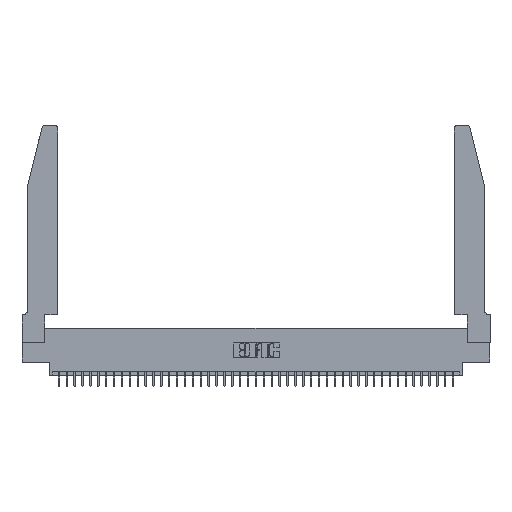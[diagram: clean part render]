
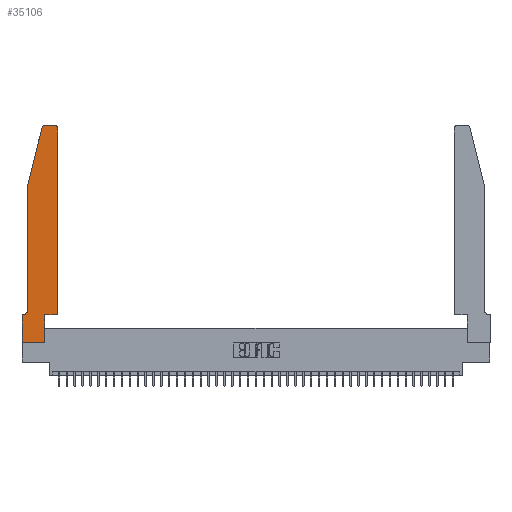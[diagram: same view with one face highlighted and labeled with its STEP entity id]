
A CAD part, top view. The second image highlights one B-rep face of the part: STEP entity #35106.
In plain terms, the highlighted planar face has unit normal (0, 0, 1).
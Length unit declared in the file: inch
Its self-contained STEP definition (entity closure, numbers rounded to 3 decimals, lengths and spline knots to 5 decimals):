
#385 = CARTESIAN_POINT ( 'NONE',  ( 0.2865, 0., 0.37 ) ) ;
#411 = CARTESIAN_POINT ( 'NONE',  ( 0.4205, 2.72, 0.37 ) ) ;
#520 = DIRECTION ( 'NONE',  ( 0., 0., 1. ) ) ;
#677 = EDGE_CURVE ( 'NONE', #34103, #35598, #38022, .T. ) ;
#1090 = EDGE_CURVE ( 'NONE', #5369, #17566, #35626, .T. ) ;
#2582 = DIRECTION ( 'NONE',  ( -1., 0., 0. ) ) ;
#2632 = DIRECTION ( 'NONE',  ( -1., 0., 0. ) ) ;
#3723 = CARTESIAN_POINT ( 'NONE',  ( 0.4505, 0.35, 0.37 ) ) ;
#3755 = VERTEX_POINT ( 'NONE', #10312 ) ;
#3899 = VECTOR ( 'NONE', #2582, 39.37008 ) ;
#3991 = ORIENTED_EDGE ( 'NONE', *, *, #20890, .T. ) ;
#4508 = CARTESIAN_POINT ( 'NONE',  ( 0.4505, 0.35, 0.37 ) ) ;
#4546 = EDGE_CURVE ( 'NONE', #33436, #18981, #41330, .T. ) ;
#5369 = VERTEX_POINT ( 'NONE', #385 ) ;
#5561 = LINE ( 'NONE', #32865, #16286 ) ;
#5621 = EDGE_CURVE ( 'NONE', #35598, #5369, #42918, .T. ) ;
#5652 = CARTESIAN_POINT ( 'NONE',  ( 0.0755, 2., 0.37 ) ) ;
#5817 = VECTOR ( 'NONE', #32319, 39.37008 ) ;
#5860 = VERTEX_POINT ( 'NONE', #25192 ) ;
#6333 = PLANE ( 'NONE',  #38865 ) ;
#6445 = CIRCLE ( 'NONE', #29824, 0.07 ) ;
#6705 = VECTOR ( 'NONE', #22979, 39.37008 ) ;
#7182 = VECTOR ( 'NONE', #7384, 39.37008 ) ;
#7300 = ORIENTED_EDGE ( 'NONE', *, *, #5621, .T. ) ;
#7384 = DIRECTION ( 'NONE',  ( 0., 1., 0. ) ) ;
#7824 = VECTOR ( 'NONE', #28045, 39.37008 ) ;
#8460 = DIRECTION ( 'NONE',  ( 1., 0., 0. ) ) ;
#8964 = ORIENTED_EDGE ( 'NONE', *, *, #19388, .T. ) ;
#9311 = VECTOR ( 'NONE', #20646, 39.37008 ) ;
#9791 = LINE ( 'NONE', #19997, #9311 ) ;
#10312 = CARTESIAN_POINT ( 'NONE',  ( 0.25487, 2.72718, 0.37 ) ) ;
#10356 = VERTEX_POINT ( 'NONE', #19273 ) ;
#11798 = LINE ( 'NONE', #25353, #39846 ) ;
#11948 = ORIENTED_EDGE ( 'NONE', *, *, #40208, .T. ) ;
#12158 = ORIENTED_EDGE ( 'NONE', *, *, #1090, .T. ) ;
#12592 = CARTESIAN_POINT ( 'NONE',  ( 0.0055, 0.42, 0.37 ) ) ;
#12982 = LINE ( 'NONE', #26535, #6705 ) ;
#14249 = DIRECTION ( 'NONE',  ( 1., 0., 0. ) ) ;
#14704 = CARTESIAN_POINT ( 'NONE',  ( 0., 0., 0.37 ) ) ;
#16005 = DIRECTION ( 'NONE',  ( -0.239, -0.971, 0. ) ) ;
#16286 = VECTOR ( 'NONE', #16005, 39.37008 ) ;
#17566 = VERTEX_POINT ( 'NONE', #32628 ) ;
#17764 = VECTOR ( 'NONE', #18122, 39.37008 ) ;
#18122 = DIRECTION ( 'NONE',  ( 0., 1., 0. ) ) ;
#18557 = ORIENTED_EDGE ( 'NONE', *, *, #677, .T. ) ;
#18661 = FACE_OUTER_BOUND ( 'NONE', #30110, .T. ) ;
#18782 = CARTESIAN_POINT ( 'NONE',  ( 0.2865, 0.35, 0.37 ) ) ;
#18981 = VERTEX_POINT ( 'NONE', #43020 ) ;
#19273 = CARTESIAN_POINT ( 'NONE',  ( 0.0755, 0.42, 0.37 ) ) ;
#19388 = EDGE_CURVE ( 'NONE', #10356, #26324, #6445, .T. ) ;
#19410 = CARTESIAN_POINT ( 'NONE',  ( 0.0755, 0.35, 0.37 ) ) ;
#19882 = CARTESIAN_POINT ( 'NONE',  ( 0., 0.35, 0.37 ) ) ;
#19997 = CARTESIAN_POINT ( 'NONE',  ( 0.2605, 2.75, 0.37 ) ) ;
#20646 = DIRECTION ( 'NONE',  ( -1., 0., 0. ) ) ;
#20683 = ORIENTED_EDGE ( 'NONE', *, *, #4546, .T. ) ;
#20890 = EDGE_CURVE ( 'NONE', #18981, #5860, #39754, .T. ) ;
#21616 = CARTESIAN_POINT ( 'NONE',  ( 0.284, 2.75, 0.37 ) ) ;
#22564 = EDGE_CURVE ( 'NONE', #17566, #33436, #11798, .T. ) ;
#22979 = DIRECTION ( 'NONE',  ( 0., -1., 0. ) ) ;
#23001 = AXIS2_PLACEMENT_3D ( 'NONE', #30895, #520, #14249 ) ;
#25192 = CARTESIAN_POINT ( 'NONE',  ( 0.4205, 2.75, 0.37 ) ) ;
#25353 = CARTESIAN_POINT ( 'NONE',  ( 0.4505, 0.35, 0.37 ) ) ;
#26324 = VERTEX_POINT ( 'NONE', #28444 ) ;
#26521 = CIRCLE ( 'NONE', #23001, 0.03 ) ;
#26535 = CARTESIAN_POINT ( 'NONE',  ( 0.0755, 2., 0.37 ) ) ;
#26592 = DIRECTION ( 'NONE',  ( 0., 0., -1. ) ) ;
#27272 = EDGE_CURVE ( 'NONE', #27278, #10356, #12982, .T. ) ;
#27278 = VERTEX_POINT ( 'NONE', #5652 ) ;
#27321 = EDGE_CURVE ( 'NONE', #26324, #34103, #35855, .T. ) ;
#28045 = DIRECTION ( 'NONE',  ( 0., -1., 0. ) ) ;
#28444 = CARTESIAN_POINT ( 'NONE',  ( 0.0055, 0.35, 0.37 ) ) ;
#29199 = CARTESIAN_POINT ( 'NONE',  ( 0., 0., 0.37 ) ) ;
#29824 = AXIS2_PLACEMENT_3D ( 'NONE', #12592, #26592, #2632 ) ;
#29977 = EDGE_CURVE ( 'NONE', #35822, #3755, #26521, .T. ) ;
#30088 = DIRECTION ( 'NONE',  ( 1., 0., 0. ) ) ;
#30110 = EDGE_LOOP ( 'NONE', ( #11948, #43516, #31095, #33142, #8964, #39483, #18557, #7300, #12158, #33891, #20683, #3991 ) ) ;
#30782 = DIRECTION ( 'NONE',  ( 1., 0., 0. ) ) ;
#30895 = CARTESIAN_POINT ( 'NONE',  ( 0.284, 2.72, 0.37 ) ) ;
#31095 = ORIENTED_EDGE ( 'NONE', *, *, #38767, .T. ) ;
#32319 = DIRECTION ( 'NONE',  ( 1., 0., 0. ) ) ;
#32628 = CARTESIAN_POINT ( 'NONE',  ( 0.2865, 0.35, 0.37 ) ) ;
#32865 = CARTESIAN_POINT ( 'NONE',  ( 0.0755, 2., 0.37 ) ) ;
#32919 = CARTESIAN_POINT ( 'NONE',  ( 0., 0.35, 0.37 ) ) ;
#33142 = ORIENTED_EDGE ( 'NONE', *, *, #27272, .T. ) ;
#33413 = DIRECTION ( 'NONE',  ( 0., 0., 1. ) ) ;
#33436 = VERTEX_POINT ( 'NONE', #3723 ) ;
#33891 = ORIENTED_EDGE ( 'NONE', *, *, #22564, .T. ) ;
#34103 = VERTEX_POINT ( 'NONE', #32919 ) ;
#34105 = DIRECTION ( 'NONE',  ( 0., 0., 1. ) ) ;
#35106 = ADVANCED_FACE ( 'NONE', ( #18661 ), #6333, .T. ) ;
#35598 = VERTEX_POINT ( 'NONE', #36030 ) ;
#35626 = LINE ( 'NONE', #18782, #17764 ) ;
#35822 = VERTEX_POINT ( 'NONE', #21616 ) ;
#35855 = LINE ( 'NONE', #19410, #3899 ) ;
#36030 = CARTESIAN_POINT ( 'NONE',  ( 0., 0., 0.37 ) ) ;
#38022 = LINE ( 'NONE', #14704, #7824 ) ;
#38767 = EDGE_CURVE ( 'NONE', #3755, #27278, #5561, .T. ) ;
#38865 = AXIS2_PLACEMENT_3D ( 'NONE', #19882, #33413, #30088 ) ;
#39483 = ORIENTED_EDGE ( 'NONE', *, *, #27321, .T. ) ;
#39754 = CIRCLE ( 'NONE', #41155, 0.03 ) ;
#39846 = VECTOR ( 'NONE', #8460, 39.37008 ) ;
#40208 = EDGE_CURVE ( 'NONE', #5860, #35822, #9791, .T. ) ;
#41155 = AXIS2_PLACEMENT_3D ( 'NONE', #411, #34105, #30782 ) ;
#41330 = LINE ( 'NONE', #4508, #7182 ) ;
#42918 = LINE ( 'NONE', #29199, #5817 ) ;
#43020 = CARTESIAN_POINT ( 'NONE',  ( 0.4505, 2.72, 0.37 ) ) ;
#43516 = ORIENTED_EDGE ( 'NONE', *, *, #29977, .T. ) ;
